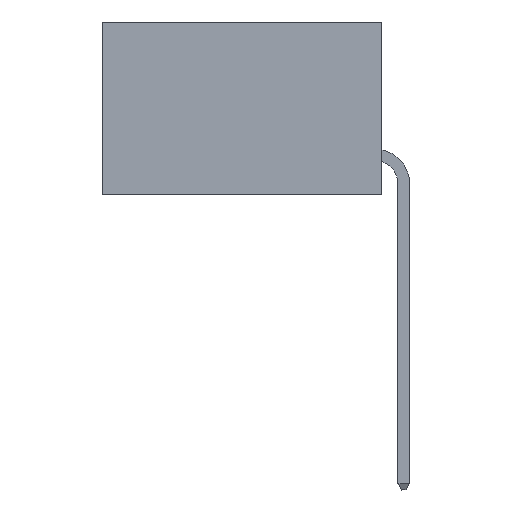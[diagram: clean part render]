
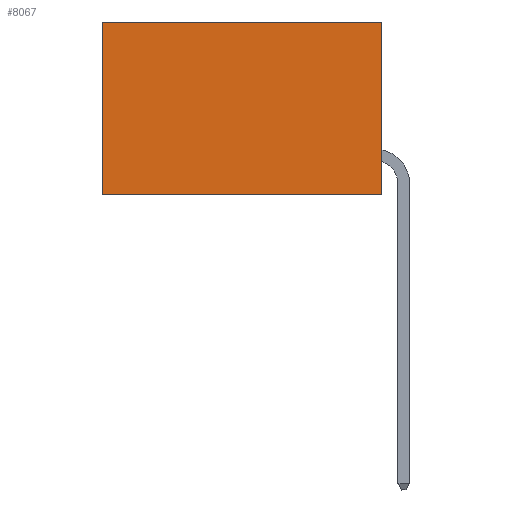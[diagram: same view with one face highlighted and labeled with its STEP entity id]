
A CAD part, left-side view. The second image highlights one B-rep face of the part: STEP entity #8067.
In plain terms, the highlighted planar face has unit normal (-1, 0, 0).
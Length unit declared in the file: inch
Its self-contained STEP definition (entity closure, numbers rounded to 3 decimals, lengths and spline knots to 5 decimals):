
#152 = ORIENTED_EDGE ( 'NONE', *, *, #23360, .F. ) ;
#481 = VERTEX_POINT ( 'NONE', #1430 ) ;
#1430 = CARTESIAN_POINT ( 'NONE',  ( 0.2875, 0.6, 0. ) ) ;
#1711 = CARTESIAN_POINT ( 'NONE',  ( 0.2875, 0., 0. ) ) ;
#1829 = DIRECTION ( 'NONE',  ( 0., 0., -1. ) ) ;
#2270 = CARTESIAN_POINT ( 'NONE',  ( 0.2875, 0., 0. ) ) ;
#4041 = CARTESIAN_POINT ( 'NONE',  ( 0.2875, 0., 0. ) ) ;
#5880 = CARTESIAN_POINT ( 'NONE',  ( 0.2875, 0., -0.37 ) ) ;
#6200 = AXIS2_PLACEMENT_3D ( 'NONE', #2270, #6220, #23960 ) ;
#6220 = DIRECTION ( 'NONE',  ( 1., 0., 0. ) ) ;
#6424 = LINE ( 'NONE', #1711, #19262 ) ;
#6669 = EDGE_CURVE ( 'NONE', #20499, #21310, #6424, .T. ) ;
#8058 = PLANE ( 'NONE',  #6200 ) ;
#8067 = ADVANCED_FACE ( 'NONE', ( #21026 ), #8058, .F. ) ;
#9231 = CARTESIAN_POINT ( 'NONE',  ( 0.2875, 0., 0. ) ) ;
#9868 = VERTEX_POINT ( 'NONE', #22582 ) ;
#11658 = ORIENTED_EDGE ( 'NONE', *, *, #20257, .T. ) ;
#13373 = ORIENTED_EDGE ( 'NONE', *, *, #18622, .T. ) ;
#13947 = CARTESIAN_POINT ( 'NONE',  ( 0.2875, 0.6, 0. ) ) ;
#14473 = VECTOR ( 'NONE', #17816, 39.37008 ) ;
#17045 = VECTOR ( 'NONE', #1829, 39.37008 ) ;
#17227 = DIRECTION ( 'NONE',  ( 0., 0., -1. ) ) ;
#17816 = DIRECTION ( 'NONE',  ( 0., 1., 0. ) ) ;
#18078 = VECTOR ( 'NONE', #24181, 39.37008 ) ;
#18622 = EDGE_CURVE ( 'NONE', #20499, #481, #21238, .T. ) ;
#19262 = VECTOR ( 'NONE', #17227, 39.37008 ) ;
#19483 = EDGE_LOOP ( 'NONE', ( #11658, #152, #21894, #13373 ) ) ;
#20257 = EDGE_CURVE ( 'NONE', #481, #9868, #25523, .T. ) ;
#20499 = VERTEX_POINT ( 'NONE', #9231 ) ;
#21026 = FACE_OUTER_BOUND ( 'NONE', #19483, .T. ) ;
#21238 = LINE ( 'NONE', #4041, #18078 ) ;
#21310 = VERTEX_POINT ( 'NONE', #25259 ) ;
#21894 = ORIENTED_EDGE ( 'NONE', *, *, #6669, .F. ) ;
#22582 = CARTESIAN_POINT ( 'NONE',  ( 0.2875, 0.6, -0.37 ) ) ;
#23360 = EDGE_CURVE ( 'NONE', #21310, #9868, #24842, .T. ) ;
#23960 = DIRECTION ( 'NONE',  ( 0., 0., -1. ) ) ;
#24181 = DIRECTION ( 'NONE',  ( 0., 1., 0. ) ) ;
#24842 = LINE ( 'NONE', #5880, #14473 ) ;
#25259 = CARTESIAN_POINT ( 'NONE',  ( 0.2875, 0., -0.37 ) ) ;
#25523 = LINE ( 'NONE', #13947, #17045 ) ;
